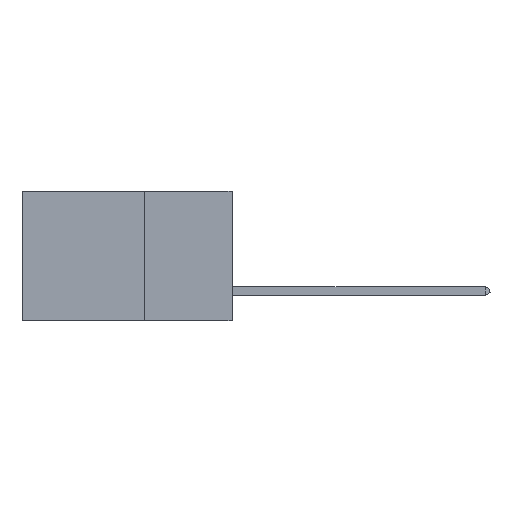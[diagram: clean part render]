
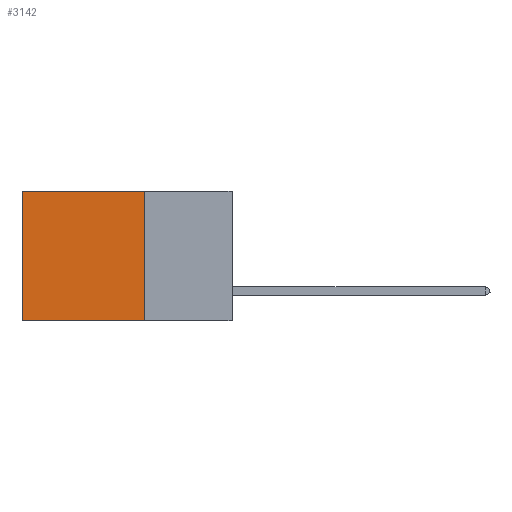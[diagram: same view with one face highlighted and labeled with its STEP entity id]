
A CAD part, left-side view. The second image highlights one B-rep face of the part: STEP entity #3142.
In plain terms, the highlighted planar face has unit normal (-1, 0, 0).
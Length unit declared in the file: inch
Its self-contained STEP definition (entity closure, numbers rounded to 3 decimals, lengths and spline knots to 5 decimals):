
#932 = EDGE_CURVE ( 'NONE', #2086, #5085, #10217, .T. ) ;
#999 = DIRECTION ( 'NONE',  ( 0., 0., -1. ) ) ;
#1550 = EDGE_CURVE ( 'NONE', #3180, #7732, #17078, .T. ) ;
#1657 = CARTESIAN_POINT ( 'NONE',  ( 0.2875, 0.6, 0. ) ) ;
#2086 = VERTEX_POINT ( 'NONE', #1657 ) ;
#2448 = FACE_OUTER_BOUND ( 'NONE', #6470, .T. ) ;
#2724 = CARTESIAN_POINT ( 'NONE',  ( 0.2875, 0.25, 0. ) ) ;
#3142 = ADVANCED_FACE ( 'NONE', ( #2448 ), #10670, .F. ) ;
#3180 = VERTEX_POINT ( 'NONE', #4205 ) ;
#4205 = CARTESIAN_POINT ( 'NONE',  ( 0.2875, 0.25, 0. ) ) ;
#4269 = CARTESIAN_POINT ( 'NONE',  ( 0.2875, 0.25, -0.37 ) ) ;
#5036 = LINE ( 'NONE', #2724, #17119 ) ;
#5085 = VERTEX_POINT ( 'NONE', #6219 ) ;
#5239 = CARTESIAN_POINT ( 'NONE',  ( 0.2875, 0.6, 0. ) ) ;
#5671 = EDGE_CURVE ( 'NONE', #7732, #5085, #13821, .T. ) ;
#6219 = CARTESIAN_POINT ( 'NONE',  ( 0.2875, 0.6, -0.37 ) ) ;
#6301 = VECTOR ( 'NONE', #12317, 39.37008 ) ;
#6470 = EDGE_LOOP ( 'NONE', ( #14269, #9644, #10360, #13928 ) ) ;
#6562 = DIRECTION ( 'NONE',  ( 0., 0., -1. ) ) ;
#6817 = DIRECTION ( 'NONE',  ( 1., 0., 0. ) ) ;
#7732 = VERTEX_POINT ( 'NONE', #14439 ) ;
#8550 = VECTOR ( 'NONE', #999, 39.37008 ) ;
#9395 = DIRECTION ( 'NONE',  ( 0., 1., 0. ) ) ;
#9644 = ORIENTED_EDGE ( 'NONE', *, *, #5671, .F. ) ;
#10217 = LINE ( 'NONE', #5239, #11056 ) ;
#10360 = ORIENTED_EDGE ( 'NONE', *, *, #1550, .F. ) ;
#10670 = PLANE ( 'NONE',  #12141 ) ;
#10904 = DIRECTION ( 'NONE',  ( 0., 0., -1. ) ) ;
#11056 = VECTOR ( 'NONE', #6562, 39.37008 ) ;
#12012 = CARTESIAN_POINT ( 'NONE',  ( 0.2875, 0.25, 0. ) ) ;
#12141 = AXIS2_PLACEMENT_3D ( 'NONE', #12012, #6817, #10904 ) ;
#12317 = DIRECTION ( 'NONE',  ( 0., 1., 0. ) ) ;
#13821 = LINE ( 'NONE', #4269, #6301 ) ;
#13928 = ORIENTED_EDGE ( 'NONE', *, *, #17046, .T. ) ;
#14269 = ORIENTED_EDGE ( 'NONE', *, *, #932, .T. ) ;
#14439 = CARTESIAN_POINT ( 'NONE',  ( 0.2875, 0.25, -0.37 ) ) ;
#15769 = CARTESIAN_POINT ( 'NONE',  ( 0.2875, 0.25, 0. ) ) ;
#17046 = EDGE_CURVE ( 'NONE', #3180, #2086, #5036, .T. ) ;
#17078 = LINE ( 'NONE', #15769, #8550 ) ;
#17119 = VECTOR ( 'NONE', #9395, 39.37008 ) ;
